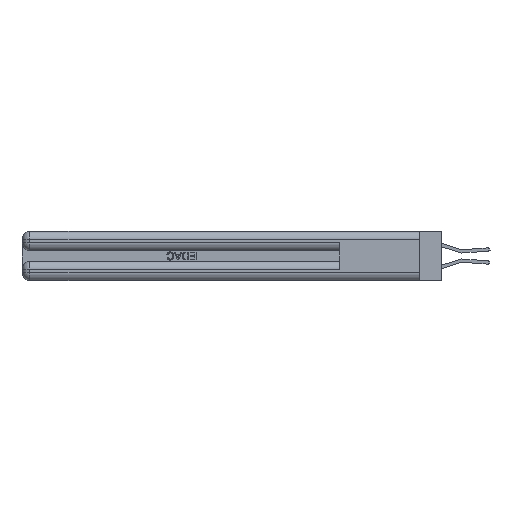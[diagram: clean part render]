
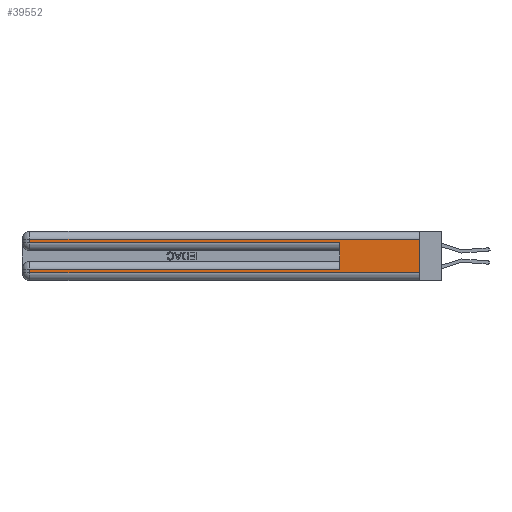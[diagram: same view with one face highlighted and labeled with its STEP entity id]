
A CAD part, left-side view. The second image highlights one B-rep face of the part: STEP entity #39552.
In plain terms, the highlighted planar face has unit normal (-1, 0, 0).
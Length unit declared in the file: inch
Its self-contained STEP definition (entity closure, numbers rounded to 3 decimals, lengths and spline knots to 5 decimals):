
#320 = EDGE_CURVE ( 'NONE', #3373, #7830, #35867, .T. ) ;
#542 = EDGE_CURVE ( 'NONE', #16541, #7151, #29856, .T. ) ;
#1212 = DIRECTION ( 'NONE',  ( 0., 0., -1. ) ) ;
#3223 = CARTESIAN_POINT ( 'NONE',  ( 0., 2.94, 0.31 ) ) ;
#3373 = VERTEX_POINT ( 'NONE', #9343 ) ;
#3381 = ORIENTED_EDGE ( 'NONE', *, *, #320, .F. ) ;
#3588 = DIRECTION ( 'NONE',  ( 1., 0., 0. ) ) ;
#3754 = ORIENTED_EDGE ( 'NONE', *, *, #4200, .T. ) ;
#4200 = EDGE_CURVE ( 'NONE', #32054, #27361, #25106, .T. ) ;
#4662 = CARTESIAN_POINT ( 'NONE',  ( 0., 2.94, 0.37 ) ) ;
#6145 = LINE ( 'NONE', #29697, #23026 ) ;
#6328 = CARTESIAN_POINT ( 'NONE',  ( 0., 0.6, 0.145 ) ) ;
#6346 = DIRECTION ( 'NONE',  ( 0., 0., -1. ) ) ;
#7151 = VERTEX_POINT ( 'NONE', #40271 ) ;
#7830 = VERTEX_POINT ( 'NONE', #33613 ) ;
#8639 = CARTESIAN_POINT ( 'NONE',  ( 0., 0., 0.31 ) ) ;
#9343 = CARTESIAN_POINT ( 'NONE',  ( 0., 0.6, 0.085 ) ) ;
#9454 = LINE ( 'NONE', #13456, #30273 ) ;
#9513 = DIRECTION ( 'NONE',  ( 0., -1., 0. ) ) ;
#9523 = DIRECTION ( 'NONE',  ( 0., 0., 1. ) ) ;
#10527 = EDGE_CURVE ( 'NONE', #7151, #28828, #26964, .T. ) ;
#11288 = AXIS2_PLACEMENT_3D ( 'NONE', #22591, #3588, #6346 ) ;
#11570 = EDGE_CURVE ( 'NONE', #28925, #7830, #36335, .T. ) ;
#12618 = ORIENTED_EDGE ( 'NONE', *, *, #542, .T. ) ;
#13456 = CARTESIAN_POINT ( 'NONE',  ( 0., 0., 0.37 ) ) ;
#13900 = VECTOR ( 'NONE', #16647, 39.37008 ) ;
#14062 = VECTOR ( 'NONE', #9523, 39.37008 ) ;
#16056 = VECTOR ( 'NONE', #9513, 39.37008 ) ;
#16111 = CARTESIAN_POINT ( 'NONE',  ( 0., 0., 0.085 ) ) ;
#16541 = VERTEX_POINT ( 'NONE', #24619 ) ;
#16647 = DIRECTION ( 'NONE',  ( 0., 1., 0. ) ) ;
#18699 = CARTESIAN_POINT ( 'NONE',  ( 0., 0., 0.06 ) ) ;
#19142 = CARTESIAN_POINT ( 'NONE',  ( 0., 0., 0.31 ) ) ;
#19465 = CARTESIAN_POINT ( 'NONE',  ( 0., 0., 0.285 ) ) ;
#21146 = EDGE_CURVE ( 'NONE', #3373, #16541, #24798, .T. ) ;
#22465 = ORIENTED_EDGE ( 'NONE', *, *, #37054, .T. ) ;
#22591 = CARTESIAN_POINT ( 'NONE',  ( 0., 0., 0.37 ) ) ;
#23026 = VECTOR ( 'NONE', #1212, 39.37008 ) ;
#23240 = DIRECTION ( 'NONE',  ( 0., 0., -1. ) ) ;
#24617 = CARTESIAN_POINT ( 'NONE',  ( 0., 0., 0.06 ) ) ;
#24618 = DIRECTION ( 'NONE',  ( 0., 1., 0. ) ) ;
#24619 = CARTESIAN_POINT ( 'NONE',  ( 0., 2.94, 0.085 ) ) ;
#24798 = LINE ( 'NONE', #16111, #13900 ) ;
#25011 = EDGE_LOOP ( 'NONE', ( #37153, #3754, #22465, #37176, #3381, #33199, #12618, #32475 ) ) ;
#25106 = LINE ( 'NONE', #8639, #27086 ) ;
#25296 = CARTESIAN_POINT ( 'NONE',  ( 0., 2.94, 0.285 ) ) ;
#26964 = LINE ( 'NONE', #18699, #16056 ) ;
#27086 = VECTOR ( 'NONE', #24618, 39.37008 ) ;
#27361 = VERTEX_POINT ( 'NONE', #3223 ) ;
#28449 = DIRECTION ( 'NONE',  ( 0., -1., 0. ) ) ;
#28828 = VERTEX_POINT ( 'NONE', #24617 ) ;
#28853 = VECTOR ( 'NONE', #23240, 39.37008 ) ;
#28925 = VERTEX_POINT ( 'NONE', #25296 ) ;
#29697 = CARTESIAN_POINT ( 'NONE',  ( 0., 2.94, 0.37 ) ) ;
#29856 = LINE ( 'NONE', #4662, #28853 ) ;
#30273 = VECTOR ( 'NONE', #35655, 39.37008 ) ;
#32054 = VERTEX_POINT ( 'NONE', #19142 ) ;
#32475 = ORIENTED_EDGE ( 'NONE', *, *, #10527, .T. ) ;
#33199 = ORIENTED_EDGE ( 'NONE', *, *, #21146, .T. ) ;
#33613 = CARTESIAN_POINT ( 'NONE',  ( 0., 0.6, 0.285 ) ) ;
#35655 = DIRECTION ( 'NONE',  ( 0., 0., -1. ) ) ;
#35867 = LINE ( 'NONE', #6328, #14062 ) ;
#36335 = LINE ( 'NONE', #19465, #38294 ) ;
#37054 = EDGE_CURVE ( 'NONE', #27361, #28925, #6145, .T. ) ;
#37153 = ORIENTED_EDGE ( 'NONE', *, *, #39147, .F. ) ;
#37176 = ORIENTED_EDGE ( 'NONE', *, *, #11570, .T. ) ;
#38294 = VECTOR ( 'NONE', #28449, 39.37008 ) ;
#38486 = PLANE ( 'NONE',  #11288 ) ;
#39147 = EDGE_CURVE ( 'NONE', #32054, #28828, #9454, .T. ) ;
#39552 = ADVANCED_FACE ( 'NONE', ( #39664 ), #38486, .F. ) ;
#39664 = FACE_OUTER_BOUND ( 'NONE', #25011, .T. ) ;
#40271 = CARTESIAN_POINT ( 'NONE',  ( 0., 2.94, 0.06 ) ) ;
